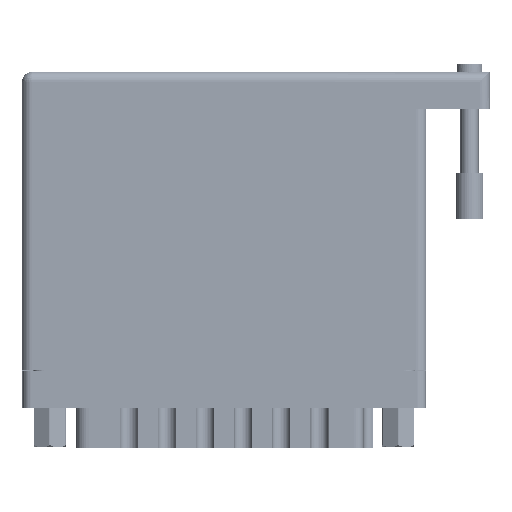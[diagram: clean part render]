
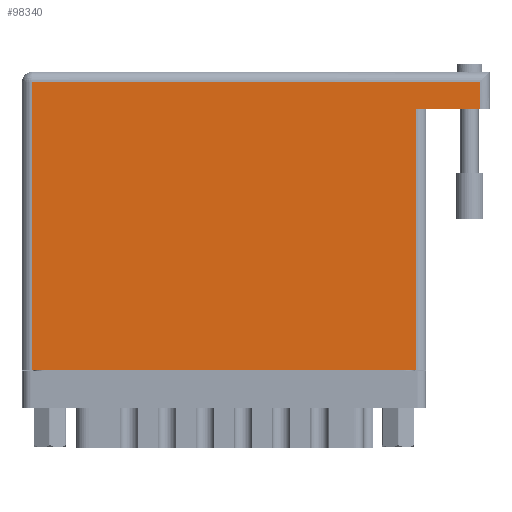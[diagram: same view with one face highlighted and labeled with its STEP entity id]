
A CAD part, front view. The second image highlights one B-rep face of the part: STEP entity #98340.
In plain terms, the highlighted face is planar.
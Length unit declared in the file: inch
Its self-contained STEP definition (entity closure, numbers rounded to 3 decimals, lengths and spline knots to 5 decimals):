
#5290 = ORIENTED_EDGE ( 'NONE', *, *, #56556, .T. ) ;
#9065 = VECTOR ( 'NONE', #41399, 39.37008 ) ;
#10177 = DIRECTION ( 'NONE',  ( -1., 0., 0. ) ) ;
#10504 = DIRECTION ( 'NONE',  ( -1., 0., 0. ) ) ;
#10873 = VECTOR ( 'NONE', #91479, 39.37008 ) ;
#11659 = FACE_OUTER_BOUND ( 'NONE', #98386, .T. ) ;
#13458 = LINE ( 'NONE', #19219, #10873 ) ;
#17186 = VERTEX_POINT ( 'NONE', #40613 ) ;
#19219 = CARTESIAN_POINT ( 'NONE',  ( 2.685, 1.774, 0. ) ) ;
#21589 = CARTESIAN_POINT ( 'NONE',  ( 3.12, 2.03, 0. ) ) ;
#21666 = VECTOR ( 'NONE', #105272, 39.37008 ) ;
#23318 = VECTOR ( 'NONE', #104706, 39.37008 ) ;
#24824 = ORIENTED_EDGE ( 'NONE', *, *, #98905, .T. ) ;
#28276 = CARTESIAN_POINT ( 'NONE',  ( 3.12, 1.96, 0. ) ) ;
#30126 = ORIENTED_EDGE ( 'NONE', *, *, #69762, .T. ) ;
#34167 = VERTEX_POINT ( 'NONE', #51761 ) ;
#34690 = CARTESIAN_POINT ( 'NONE',  ( 2.685, 1.774, 0. ) ) ;
#38142 = VECTOR ( 'NONE', #79921, 39.37008 ) ;
#38346 = LINE ( 'NONE', #56146, #23318 ) ;
#40613 = CARTESIAN_POINT ( 'NONE',  ( 2.685, 0., 0. ) ) ;
#41293 = EDGE_CURVE ( 'NONE', #88253, #51506, #104770, .T. ) ;
#41399 = DIRECTION ( 'NONE',  ( 1., 0., 0. ) ) ;
#43043 = PLANE ( 'NONE',  #45382 ) ;
#45382 = AXIS2_PLACEMENT_3D ( 'NONE', #99901, #75656, #10177 ) ;
#51506 = VERTEX_POINT ( 'NONE', #81939 ) ;
#51761 = CARTESIAN_POINT ( 'NONE',  ( 0.07, 0., 0. ) ) ;
#52195 = CARTESIAN_POINT ( 'NONE',  ( 3.12, 1.774, 0. ) ) ;
#56146 = CARTESIAN_POINT ( 'NONE',  ( 0.07, 0., 0. ) ) ;
#56556 = EDGE_CURVE ( 'NONE', #17186, #73806, #13458, .T. ) ;
#59935 = EDGE_CURVE ( 'NONE', #86683, #73806, #102238, .T. ) ;
#61172 = ORIENTED_EDGE ( 'NONE', *, *, #41293, .T. ) ;
#61565 = LINE ( 'NONE', #98596, #9065 ) ;
#69157 = EDGE_CURVE ( 'NONE', #51506, #34167, #38346, .T. ) ;
#69762 = EDGE_CURVE ( 'NONE', #86683, #88253, #85602, .T. ) ;
#73806 = VERTEX_POINT ( 'NONE', #34690 ) ;
#75656 = DIRECTION ( 'NONE',  ( 0., 0., -1. ) ) ;
#79921 = DIRECTION ( 'NONE',  ( 0., 1., 0. ) ) ;
#81904 = VECTOR ( 'NONE', #10504, 39.37008 ) ;
#81939 = CARTESIAN_POINT ( 'NONE',  ( 0.07, 1.96, 0. ) ) ;
#82975 = ORIENTED_EDGE ( 'NONE', *, *, #69157, .T. ) ;
#85602 = LINE ( 'NONE', #21589, #38142 ) ;
#86683 = VERTEX_POINT ( 'NONE', #52195 ) ;
#88253 = VERTEX_POINT ( 'NONE', #28276 ) ;
#90286 = CARTESIAN_POINT ( 'NONE',  ( 3.19, 1.774, 0. ) ) ;
#91479 = DIRECTION ( 'NONE',  ( 0., 1., 0. ) ) ;
#94604 = ORIENTED_EDGE ( 'NONE', *, *, #59935, .F. ) ;
#98340 = ADVANCED_FACE ( 'NONE', ( #11659 ), #43043, .F. ) ;
#98386 = EDGE_LOOP ( 'NONE', ( #24824, #5290, #94604, #30126, #61172, #82975 ) ) ;
#98596 = CARTESIAN_POINT ( 'NONE',  ( 0., 0., 0. ) ) ;
#98905 = EDGE_CURVE ( 'NONE', #34167, #17186, #61565, .T. ) ;
#99513 = CARTESIAN_POINT ( 'NONE',  ( 0., 1.96, 0. ) ) ;
#99901 = CARTESIAN_POINT ( 'NONE',  ( 0., 2.03, 0. ) ) ;
#102238 = LINE ( 'NONE', #90286, #21666 ) ;
#104706 = DIRECTION ( 'NONE',  ( 0., -1., 0. ) ) ;
#104770 = LINE ( 'NONE', #99513, #81904 ) ;
#105272 = DIRECTION ( 'NONE',  ( -1., 0., 0. ) ) ;
